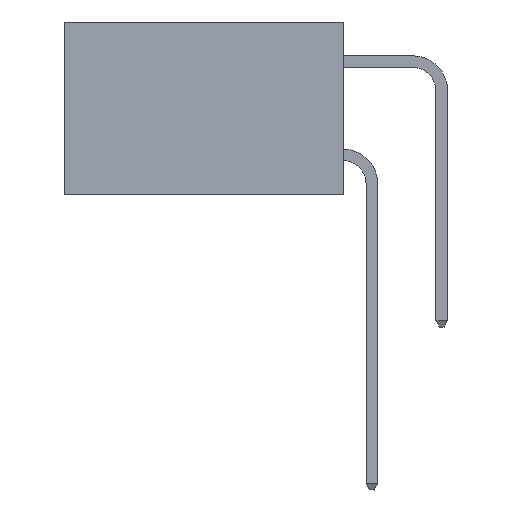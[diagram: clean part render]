
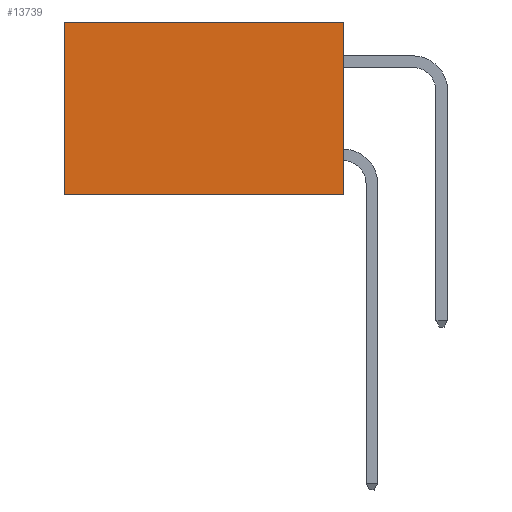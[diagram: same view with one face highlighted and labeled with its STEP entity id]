
A CAD part, left-side view. The second image highlights one B-rep face of the part: STEP entity #13739.
In plain terms, the highlighted planar face has unit normal (-1, 0, 0).
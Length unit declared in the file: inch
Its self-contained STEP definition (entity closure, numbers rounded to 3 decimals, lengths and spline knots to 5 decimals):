
#2255 = FACE_OUTER_BOUND ( 'NONE', #10061, .T. ) ;
#2421 = CARTESIAN_POINT ( 'NONE',  ( 0.2615, 0., 0. ) ) ;
#3181 = CARTESIAN_POINT ( 'NONE',  ( 0.2615, 0., -0.37 ) ) ;
#4487 = ORIENTED_EDGE ( 'NONE', *, *, #14720, .F. ) ;
#4759 = AXIS2_PLACEMENT_3D ( 'NONE', #7460, #8127, #22501 ) ;
#5310 = DIRECTION ( 'NONE',  ( 0., 1., 0. ) ) ;
#5450 = VECTOR ( 'NONE', #22673, 39.37008 ) ;
#6151 = ORIENTED_EDGE ( 'NONE', *, *, #7560, .T. ) ;
#6169 = LINE ( 'NONE', #2421, #5450 ) ;
#6886 = CARTESIAN_POINT ( 'NONE',  ( 0.2615, 0.6, 0. ) ) ;
#7436 = DIRECTION ( 'NONE',  ( 0., 0., -1. ) ) ;
#7460 = CARTESIAN_POINT ( 'NONE',  ( 0.2615, 0., -0.37 ) ) ;
#7560 = EDGE_CURVE ( 'NONE', #11669, #18463, #16044, .T. ) ;
#7699 = LINE ( 'NONE', #15900, #15931 ) ;
#8127 = DIRECTION ( 'NONE',  ( 1., 0., 0. ) ) ;
#9470 = LINE ( 'NONE', #3181, #20731 ) ;
#10061 = EDGE_LOOP ( 'NONE', ( #6151, #13485, #4487, #22240 ) ) ;
#10267 = EDGE_CURVE ( 'NONE', #22276, #11669, #6169, .T. ) ;
#11669 = VERTEX_POINT ( 'NONE', #6886 ) ;
#13485 = ORIENTED_EDGE ( 'NONE', *, *, #19974, .F. ) ;
#13515 = VECTOR ( 'NONE', #14159, 39.37008 ) ;
#13739 = ADVANCED_FACE ( 'NONE', ( #2255 ), #14314, .F. ) ;
#14159 = DIRECTION ( 'NONE',  ( 0., 0., -1. ) ) ;
#14314 = PLANE ( 'NONE',  #4759 ) ;
#14720 = EDGE_CURVE ( 'NONE', #22276, #24292, #7699, .T. ) ;
#15900 = CARTESIAN_POINT ( 'NONE',  ( 0.2615, 0., -0.37 ) ) ;
#15931 = VECTOR ( 'NONE', #7436, 39.37008 ) ;
#16044 = LINE ( 'NONE', #16439, #13515 ) ;
#16439 = CARTESIAN_POINT ( 'NONE',  ( 0.2615, 0.6, -0.37 ) ) ;
#16638 = CARTESIAN_POINT ( 'NONE',  ( 0.2615, 0., -0.37 ) ) ;
#17442 = CARTESIAN_POINT ( 'NONE',  ( 0.2615, 0., 0. ) ) ;
#18463 = VERTEX_POINT ( 'NONE', #18767 ) ;
#18767 = CARTESIAN_POINT ( 'NONE',  ( 0.2615, 0.6, -0.37 ) ) ;
#19974 = EDGE_CURVE ( 'NONE', #24292, #18463, #9470, .T. ) ;
#20731 = VECTOR ( 'NONE', #5310, 39.37008 ) ;
#22240 = ORIENTED_EDGE ( 'NONE', *, *, #10267, .T. ) ;
#22276 = VERTEX_POINT ( 'NONE', #17442 ) ;
#22501 = DIRECTION ( 'NONE',  ( 0., 0., -1. ) ) ;
#22673 = DIRECTION ( 'NONE',  ( 0., 1., 0. ) ) ;
#24292 = VERTEX_POINT ( 'NONE', #16638 ) ;
